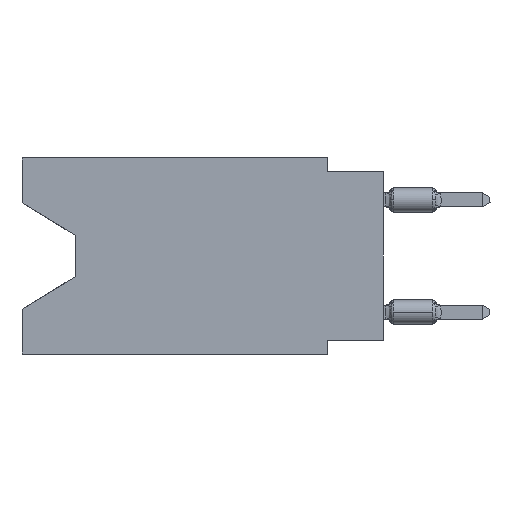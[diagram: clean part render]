
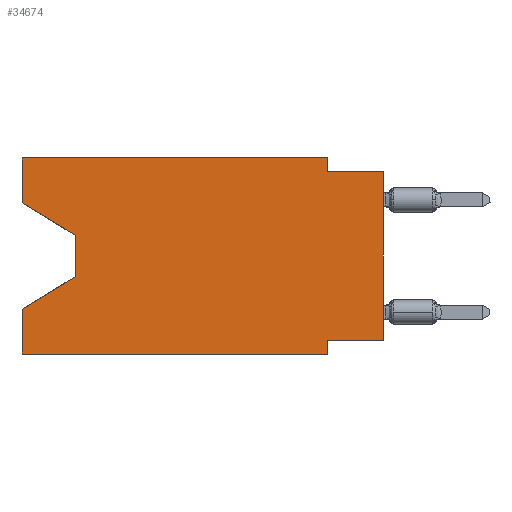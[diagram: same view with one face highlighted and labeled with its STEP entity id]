
A CAD part, left-side view. The second image highlights one B-rep face of the part: STEP entity #34674.
In plain terms, the highlighted planar face has unit normal (-1, 0, 0).
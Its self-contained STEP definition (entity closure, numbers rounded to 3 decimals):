
#37 = CARTESIAN_POINT ( 'NONE',  ( 0., 0., 0. ) ) ;
#377 = ORIENTED_EDGE ( 'NONE', *, *, #14600, .T. ) ;
#480 = VERTEX_POINT ( 'NONE', #49514 ) ;
#806 = DIRECTION ( 'NONE',  ( 0., 0., -1. ) ) ;
#1344 = CARTESIAN_POINT ( 'NONE',  ( 0., 2.54, 0. ) ) ;
#1525 = ORIENTED_EDGE ( 'NONE', *, *, #49637, .T. ) ;
#1677 = CARTESIAN_POINT ( 'NONE',  ( 0., 2.54, -0.635 ) ) ;
#2685 = VERTEX_POINT ( 'NONE', #8493 ) ;
#3098 = VECTOR ( 'NONE', #50598, 1000. ) ;
#3608 = DIRECTION ( 'NONE',  ( 0., -1., 0. ) ) ;
#3818 = LINE ( 'NONE', #20780, #3098 ) ;
#5126 = LINE ( 'NONE', #47722, #27473 ) ;
#6969 = ORIENTED_EDGE ( 'NONE', *, *, #36574, .T. ) ;
#7120 = ORIENTED_EDGE ( 'NONE', *, *, #46253, .F. ) ;
#7387 = EDGE_CURVE ( 'NONE', #44194, #14522, #13318, .T. ) ;
#7537 = VECTOR ( 'NONE', #34509, 1000. ) ;
#7699 = CARTESIAN_POINT ( 'NONE',  ( 0., 16.383, 0. ) ) ;
#8007 = ORIENTED_EDGE ( 'NONE', *, *, #54659, .F. ) ;
#8493 = CARTESIAN_POINT ( 'NONE',  ( 0., 2.54, 0. ) ) ;
#8604 = CARTESIAN_POINT ( 'NONE',  ( 0., 16.383, -8.89 ) ) ;
#9874 = VERTEX_POINT ( 'NONE', #29207 ) ;
#10608 = CARTESIAN_POINT ( 'NONE',  ( 0., 2.54, -8.89 ) ) ;
#11138 = CARTESIAN_POINT ( 'NONE',  ( 0., 16.383, 0. ) ) ;
#11645 = DIRECTION ( 'NONE',  ( 0., -1., 0. ) ) ;
#11735 = ORIENTED_EDGE ( 'NONE', *, *, #15544, .F. ) ;
#13318 = LINE ( 'NONE', #8604, #23938 ) ;
#14327 = ORIENTED_EDGE ( 'NONE', *, *, #21965, .F. ) ;
#14522 = VERTEX_POINT ( 'NONE', #10608 ) ;
#14600 = EDGE_CURVE ( 'NONE', #40823, #480, #16155, .T. ) ;
#15365 = CARTESIAN_POINT ( 'NONE',  ( 0., 13.97, -3.505 ) ) ;
#15381 = AXIS2_PLACEMENT_3D ( 'NONE', #7699, #41658, #20496 ) ;
#15544 = EDGE_CURVE ( 'NONE', #31493, #2685, #36151, .T. ) ;
#16155 = LINE ( 'NONE', #37, #36463 ) ;
#16836 = VECTOR ( 'NONE', #23617, 1000. ) ;
#16977 = ORIENTED_EDGE ( 'NONE', *, *, #7387, .T. ) ;
#18093 = LINE ( 'NONE', #21995, #7537 ) ;
#18420 = LINE ( 'NONE', #48786, #54008 ) ;
#18700 = VECTOR ( 'NONE', #11645, 1000. ) ;
#19165 = LINE ( 'NONE', #27246, #16836 ) ;
#19676 = DIRECTION ( 'NONE',  ( 0., 1., 0. ) ) ;
#20254 = ORIENTED_EDGE ( 'NONE', *, *, #54344, .F. ) ;
#20496 = DIRECTION ( 'NONE',  ( 0., 0., -1. ) ) ;
#20780 = CARTESIAN_POINT ( 'NONE',  ( 0., 16.383, -2.038 ) ) ;
#21965 = EDGE_CURVE ( 'NONE', #44194, #35594, #37008, .T. ) ;
#21995 = CARTESIAN_POINT ( 'NONE',  ( 0., 13.97, -3.505 ) ) ;
#23196 = DIRECTION ( 'NONE',  ( 0., 0., 1. ) ) ;
#23617 = DIRECTION ( 'NONE',  ( 0., -1., 0. ) ) ;
#23938 = VECTOR ( 'NONE', #3608, 1000. ) ;
#23976 = CARTESIAN_POINT ( 'NONE',  ( 0., 16.383, -6.852 ) ) ;
#24053 = ORIENTED_EDGE ( 'NONE', *, *, #51983, .F. ) ;
#24137 = LINE ( 'NONE', #27757, #34486 ) ;
#24300 = ORIENTED_EDGE ( 'NONE', *, *, #33680, .F. ) ;
#24368 = ORIENTED_EDGE ( 'NONE', *, *, #42959, .T. ) ;
#25365 = VECTOR ( 'NONE', #27190, 1000. ) ;
#25822 = VERTEX_POINT ( 'NONE', #43949 ) ;
#27190 = DIRECTION ( 'NONE',  ( 0., 0.855, -0.519 ) ) ;
#27246 = CARTESIAN_POINT ( 'NONE',  ( 0., 0., -0.635 ) ) ;
#27473 = VECTOR ( 'NONE', #23196, 1000. ) ;
#27757 = CARTESIAN_POINT ( 'NONE',  ( 0., 0., -8.255 ) ) ;
#29207 = CARTESIAN_POINT ( 'NONE',  ( 0., 2.54, -8.255 ) ) ;
#30434 = VECTOR ( 'NONE', #806, 1000. ) ;
#30790 = VERTEX_POINT ( 'NONE', #15365 ) ;
#31493 = VERTEX_POINT ( 'NONE', #34922 ) ;
#32176 = VERTEX_POINT ( 'NONE', #33154 ) ;
#33154 = CARTESIAN_POINT ( 'NONE',  ( 0., 13.97, -5.385 ) ) ;
#33578 = CARTESIAN_POINT ( 'NONE',  ( 0., 16.383, -8.89 ) ) ;
#33680 = EDGE_CURVE ( 'NONE', #2685, #44557, #47561, .T. ) ;
#34486 = VECTOR ( 'NONE', #19676, 1000. ) ;
#34509 = DIRECTION ( 'NONE',  ( 0., 0., -1. ) ) ;
#34674 = ADVANCED_FACE ( 'NONE', ( #38036 ), #54766, .F. ) ;
#34922 = CARTESIAN_POINT ( 'NONE',  ( 0., 16.383, 0. ) ) ;
#35594 = VERTEX_POINT ( 'NONE', #23976 ) ;
#35801 = LINE ( 'NONE', #52553, #25365 ) ;
#36151 = LINE ( 'NONE', #41163, #18700 ) ;
#36276 = EDGE_LOOP ( 'NONE', ( #24368, #1525, #6969, #14327, #16977, #24053, #7120, #377, #20254, #24300, #11735, #8007 ) ) ;
#36463 = VECTOR ( 'NONE', #38414, 1000. ) ;
#36574 = EDGE_CURVE ( 'NONE', #32176, #35594, #35801, .T. ) ;
#37008 = LINE ( 'NONE', #11138, #40438 ) ;
#38036 = FACE_OUTER_BOUND ( 'NONE', #36276, .T. ) ;
#38414 = DIRECTION ( 'NONE',  ( 0., 0., 1. ) ) ;
#40438 = VECTOR ( 'NONE', #40661, 1000. ) ;
#40661 = DIRECTION ( 'NONE',  ( 0., 0., 1. ) ) ;
#40823 = VERTEX_POINT ( 'NONE', #42350 ) ;
#41163 = CARTESIAN_POINT ( 'NONE',  ( 0., 16.383, 0. ) ) ;
#41658 = DIRECTION ( 'NONE',  ( 1., 0., 0. ) ) ;
#42350 = CARTESIAN_POINT ( 'NONE',  ( 0., 0., -8.255 ) ) ;
#42959 = EDGE_CURVE ( 'NONE', #25822, #30790, #3818, .T. ) ;
#43949 = CARTESIAN_POINT ( 'NONE',  ( 0., 16.383, -2.038 ) ) ;
#44194 = VERTEX_POINT ( 'NONE', #33578 ) ;
#44557 = VERTEX_POINT ( 'NONE', #1677 ) ;
#46253 = EDGE_CURVE ( 'NONE', #40823, #9874, #24137, .T. ) ;
#47561 = LINE ( 'NONE', #1344, #30434 ) ;
#47722 = CARTESIAN_POINT ( 'NONE',  ( 0., 16.383, 0. ) ) ;
#48786 = CARTESIAN_POINT ( 'NONE',  ( 0., 2.54, -8.89 ) ) ;
#49332 = DIRECTION ( 'NONE',  ( 0., 0., -1. ) ) ;
#49514 = CARTESIAN_POINT ( 'NONE',  ( 0., 0., -0.635 ) ) ;
#49637 = EDGE_CURVE ( 'NONE', #30790, #32176, #18093, .T. ) ;
#50598 = DIRECTION ( 'NONE',  ( 0., -0.855, -0.519 ) ) ;
#51983 = EDGE_CURVE ( 'NONE', #9874, #14522, #18420, .T. ) ;
#52553 = CARTESIAN_POINT ( 'NONE',  ( 0., 13.97, -5.385 ) ) ;
#54008 = VECTOR ( 'NONE', #49332, 1000. ) ;
#54344 = EDGE_CURVE ( 'NONE', #44557, #480, #19165, .T. ) ;
#54659 = EDGE_CURVE ( 'NONE', #25822, #31493, #5126, .T. ) ;
#54766 = PLANE ( 'NONE',  #15381 ) ;
